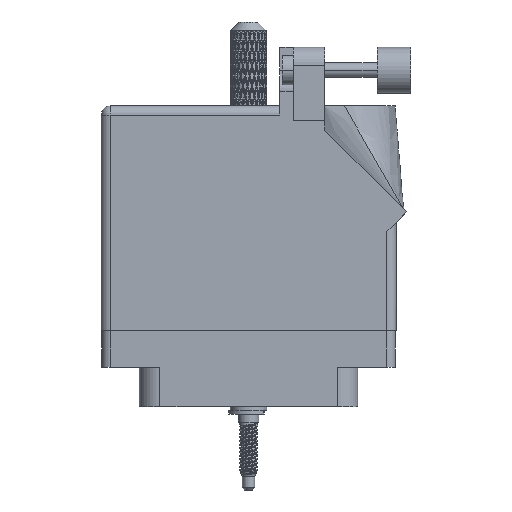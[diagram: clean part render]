
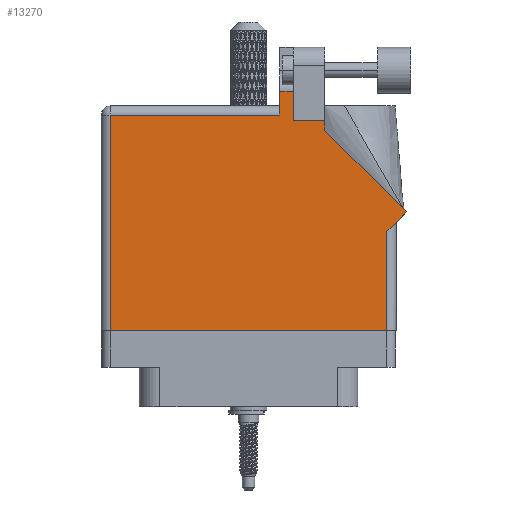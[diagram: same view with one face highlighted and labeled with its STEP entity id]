
A CAD part, front view. The second image highlights one B-rep face of the part: STEP entity #13270.
In plain terms, the highlighted face is planar.
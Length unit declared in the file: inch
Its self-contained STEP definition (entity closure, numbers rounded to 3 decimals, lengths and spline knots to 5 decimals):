
#2757 = DIRECTION ( 'NONE',  ( 0., 1., 0. ) ) ;
#3585 = VERTEX_POINT ( 'NONE', #9887 ) ;
#4522 = CARTESIAN_POINT ( 'NONE',  ( 0.212, 1.5315, 0.455 ) ) ;
#5369 = EDGE_CURVE ( 'NONE', #13275, #43560, #54915, .T. ) ;
#5617 = DIRECTION ( 'NONE',  ( -1., 0., 0. ) ) ;
#6961 = ORIENTED_EDGE ( 'NONE', *, *, #73964, .T. ) ;
#9657 = VECTOR ( 'NONE', #48426, 39.37008 ) ;
#9887 = CARTESIAN_POINT ( 'NONE',  ( 0.519, 1.33, 0.455 ) ) ;
#12732 = DIRECTION ( 'NONE',  ( 0., 1., 0. ) ) ;
#12847 = PLANE ( 'NONE',  #55477 ) ;
#13270 = ADVANCED_FACE ( 'NONE', ( #35072 ), #12847, .F. ) ;
#13275 = VERTEX_POINT ( 'NONE', #54746 ) ;
#15164 = CARTESIAN_POINT ( 'NONE',  ( 0.212, 1.43, 0.455 ) ) ;
#16055 = CARTESIAN_POINT ( 'NONE',  ( -1.005, -0.1, 0.455 ) ) ;
#21713 = DIRECTION ( 'NONE',  ( -1., 0., 0. ) ) ;
#23085 = DIRECTION ( 'NONE',  ( 0., 1., 0. ) ) ;
#23657 = LINE ( 'NONE', #55348, #71071 ) ;
#23922 = DIRECTION ( 'NONE',  ( 0., -1., 0. ) ) ;
#25174 = CARTESIAN_POINT ( 'NONE',  ( 0.212, 1.368, 0.455 ) ) ;
#25464 = EDGE_LOOP ( 'NONE', ( #94919, #64841, #6961, #70425, #88587, #99919, #34902, #65660, #105255, #44339, #32525 ) ) ;
#27155 = CARTESIAN_POINT ( 'NONE',  ( 0.943, 0.637, 0.455 ) ) ;
#27910 = VECTOR ( 'NONE', #58933, 39.37008 ) ;
#27936 = EDGE_CURVE ( 'NONE', #3585, #52916, #23657, .T. ) ;
#30879 = CARTESIAN_POINT ( 'NONE',  ( 1.07571, 0.70771, 0.455 ) ) ;
#31357 = VECTOR ( 'NONE', #41103, 39.37008 ) ;
#32525 = ORIENTED_EDGE ( 'NONE', *, *, #27936, .T. ) ;
#34902 = ORIENTED_EDGE ( 'NONE', *, *, #79897, .T. ) ;
#35072 = FACE_OUTER_BOUND ( 'NONE', #25464, .T. ) ;
#35875 = CARTESIAN_POINT ( 'NONE',  ( 0.943, 0.575, 0.455 ) ) ;
#36214 = LINE ( 'NONE', #15164, #63276 ) ;
#36622 = VECTOR ( 'NONE', #2757, 39.37008 ) ;
#37182 = CARTESIAN_POINT ( 'NONE',  ( 0.519, 1.26442, 0.455 ) ) ;
#37238 = EDGE_CURVE ( 'NONE', #49288, #76732, #45631, .T. ) ;
#38205 = DIRECTION ( 'NONE',  ( 0., 0., -1. ) ) ;
#40431 = VECTOR ( 'NONE', #23922, 39.37008 ) ;
#40513 = LINE ( 'NONE', #96548, #59793 ) ;
#41103 = DIRECTION ( 'NONE',  ( 1., 0., 0. ) ) ;
#43560 = VERTEX_POINT ( 'NONE', #4522 ) ;
#44339 = ORIENTED_EDGE ( 'NONE', *, *, #87486, .T. ) ;
#45631 = LINE ( 'NONE', #97019, #40431 ) ;
#45906 = VERTEX_POINT ( 'NONE', #59284 ) ;
#47514 = DIRECTION ( 'NONE',  ( -1., 0., 0. ) ) ;
#47711 = VERTEX_POINT ( 'NONE', #93517 ) ;
#48407 = EDGE_CURVE ( 'NONE', #81138, #47711, #52558, .T. ) ;
#48426 = DIRECTION ( 'NONE',  ( -0.707, 0.707, 0. ) ) ;
#49288 = VERTEX_POINT ( 'NONE', #87466 ) ;
#51981 = LINE ( 'NONE', #30879, #9657 ) ;
#52210 = DIRECTION ( 'NONE',  ( 0.707, 0.707, 0. ) ) ;
#52558 = LINE ( 'NONE', #93087, #89681 ) ;
#52916 = VERTEX_POINT ( 'NONE', #65474 ) ;
#54746 = CARTESIAN_POINT ( 'NONE',  ( 0.306, 1.5315, 0.455 ) ) ;
#54915 = LINE ( 'NONE', #76408, #27910 ) ;
#55348 = CARTESIAN_POINT ( 'NONE',  ( 0.519, 1.33, 0.455 ) ) ;
#55477 = AXIS2_PLACEMENT_3D ( 'NONE', #95579, #38205, #5617 ) ;
#55618 = EDGE_CURVE ( 'NONE', #102173, #49288, #98354, .T. ) ;
#57157 = LINE ( 'NONE', #27155, #36622 ) ;
#58933 = DIRECTION ( 'NONE',  ( -1., 0., 0. ) ) ;
#59284 = CARTESIAN_POINT ( 'NONE',  ( 0.943, -0.1, 0.455 ) ) ;
#59793 = VECTOR ( 'NONE', #23085, 39.37008 ) ;
#60677 = CARTESIAN_POINT ( 'NONE',  ( -0.943, -0.1, 0.455 ) ) ;
#63276 = VECTOR ( 'NONE', #72517, 39.37008 ) ;
#63684 = EDGE_CURVE ( 'NONE', #47711, #83727, #51981, .T. ) ;
#63755 = VECTOR ( 'NONE', #47514, 39.37008 ) ;
#64841 = ORIENTED_EDGE ( 'NONE', *, *, #5369, .T. ) ;
#65474 = CARTESIAN_POINT ( 'NONE',  ( 0.306, 1.33, 0.455 ) ) ;
#65660 = ORIENTED_EDGE ( 'NONE', *, *, #48407, .T. ) ;
#70425 = ORIENTED_EDGE ( 'NONE', *, *, #55618, .T. ) ;
#71071 = VECTOR ( 'NONE', #21713, 39.37008 ) ;
#72517 = DIRECTION ( 'NONE',  ( 0., -1., 0. ) ) ;
#73964 = EDGE_CURVE ( 'NONE', #43560, #102173, #36214, .T. ) ;
#76408 = CARTESIAN_POINT ( 'NONE',  ( 0.63677, 1.5315, 0.455 ) ) ;
#76732 = VERTEX_POINT ( 'NONE', #60677 ) ;
#79897 = EDGE_CURVE ( 'NONE', #45906, #81138, #57157, .T. ) ;
#81138 = VERTEX_POINT ( 'NONE', #35875 ) ;
#83727 = VERTEX_POINT ( 'NONE', #37182 ) ;
#87466 = CARTESIAN_POINT ( 'NONE',  ( -0.943, 1.368, 0.455 ) ) ;
#87486 = EDGE_CURVE ( 'NONE', #83727, #3585, #40513, .T. ) ;
#88587 = ORIENTED_EDGE ( 'NONE', *, *, #37238, .T. ) ;
#89032 = LINE ( 'NONE', #16055, #31357 ) ;
#89681 = VECTOR ( 'NONE', #52210, 39.37008 ) ;
#91662 = EDGE_CURVE ( 'NONE', #52916, #13275, #95728, .T. ) ;
#93087 = CARTESIAN_POINT ( 'NONE',  ( 1.005, 0.637, 0.455 ) ) ;
#93152 = VECTOR ( 'NONE', #12732, 39.37008 ) ;
#93517 = CARTESIAN_POINT ( 'NONE',  ( 1.07571, 0.70771, 0.455 ) ) ;
#94919 = ORIENTED_EDGE ( 'NONE', *, *, #91662, .T. ) ;
#95579 = CARTESIAN_POINT ( 'NONE',  ( -1.005, 1.43, 0.455 ) ) ;
#95728 = LINE ( 'NONE', #101171, #93152 ) ;
#96548 = CARTESIAN_POINT ( 'NONE',  ( 0.519, 1.26442, 0.455 ) ) ;
#96600 = CARTESIAN_POINT ( 'NONE',  ( -1.005, 1.368, 0.455 ) ) ;
#97019 = CARTESIAN_POINT ( 'NONE',  ( -0.943, -0.1, 0.455 ) ) ;
#98354 = LINE ( 'NONE', #96600, #63755 ) ;
#99919 = ORIENTED_EDGE ( 'NONE', *, *, #104442, .T. ) ;
#101171 = CARTESIAN_POINT ( 'NONE',  ( 0.306, 1.33, 0.455 ) ) ;
#102173 = VERTEX_POINT ( 'NONE', #25174 ) ;
#104442 = EDGE_CURVE ( 'NONE', #76732, #45906, #89032, .T. ) ;
#105255 = ORIENTED_EDGE ( 'NONE', *, *, #63684, .T. ) ;
